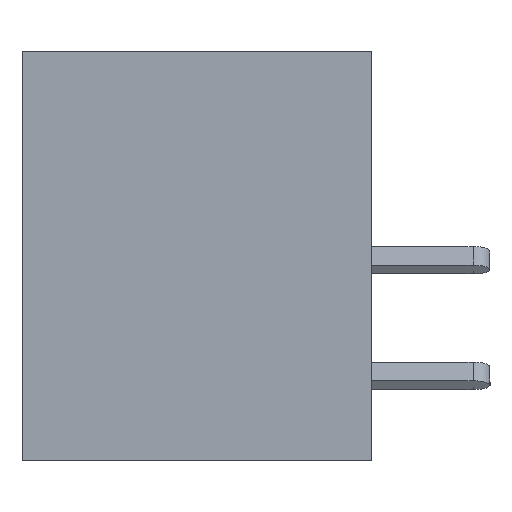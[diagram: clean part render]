
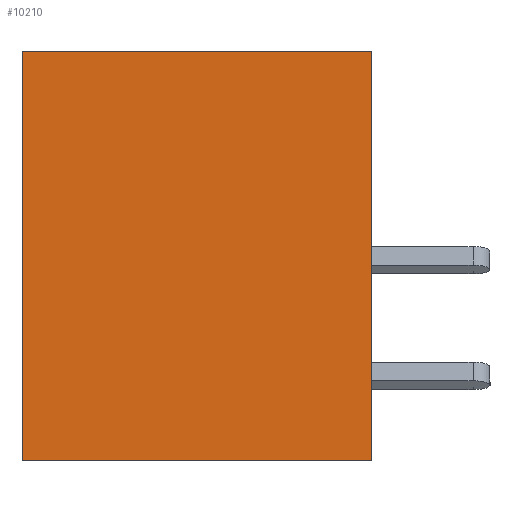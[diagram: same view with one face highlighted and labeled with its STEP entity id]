
A CAD part, left-side view. The second image highlights one B-rep face of the part: STEP entity #10210.
In plain terms, the highlighted planar face has unit normal (-1, 0, 0).
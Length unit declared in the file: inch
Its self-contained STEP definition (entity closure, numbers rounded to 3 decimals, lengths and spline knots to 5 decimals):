
#435 = VERTEX_POINT ( 'NONE', #22422 ) ;
#502 = CARTESIAN_POINT ( 'NONE',  ( 0., 0.453, 0. ) ) ;
#1654 = VECTOR ( 'NONE', #20604, 39.37008 ) ;
#2089 = DIRECTION ( 'NONE',  ( 0., 0., 1. ) ) ;
#2254 = CARTESIAN_POINT ( 'NONE',  ( 0., 0.453, 0. ) ) ;
#2281 = EDGE_CURVE ( 'NONE', #12305, #7209, #14896, .T. ) ;
#3637 = CARTESIAN_POINT ( 'NONE',  ( 0., 0.453, 0. ) ) ;
#3675 = VECTOR ( 'NONE', #17162, 39.37008 ) ;
#4034 = EDGE_CURVE ( 'NONE', #7209, #435, #6581, .T. ) ;
#5553 = DIRECTION ( 'NONE',  ( 0., 0., -1. ) ) ;
#6581 = LINE ( 'NONE', #19888, #15384 ) ;
#7209 = VERTEX_POINT ( 'NONE', #13214 ) ;
#7960 = ORIENTED_EDGE ( 'NONE', *, *, #4034, .T. ) ;
#9922 = EDGE_LOOP ( 'NONE', ( #7960, #14663, #12799, #20700 ) ) ;
#10210 = ADVANCED_FACE ( 'NONE', ( #11950 ), #14912, .F. ) ;
#10369 = VERTEX_POINT ( 'NONE', #14767 ) ;
#11029 = EDGE_CURVE ( 'NONE', #12305, #10369, #14261, .T. ) ;
#11950 = FACE_OUTER_BOUND ( 'NONE', #9922, .T. ) ;
#12305 = VERTEX_POINT ( 'NONE', #23665 ) ;
#12799 = ORIENTED_EDGE ( 'NONE', *, *, #11029, .F. ) ;
#13196 = CARTESIAN_POINT ( 'NONE',  ( 0., 0.453, -0.531 ) ) ;
#13214 = CARTESIAN_POINT ( 'NONE',  ( 0., 0., -0.531 ) ) ;
#14261 = LINE ( 'NONE', #2254, #21632 ) ;
#14663 = ORIENTED_EDGE ( 'NONE', *, *, #23825, .F. ) ;
#14767 = CARTESIAN_POINT ( 'NONE',  ( 0., 0.453, 0. ) ) ;
#14896 = LINE ( 'NONE', #13196, #1654 ) ;
#14912 = PLANE ( 'NONE',  #19265 ) ;
#15384 = VECTOR ( 'NONE', #16343, 39.37008 ) ;
#16343 = DIRECTION ( 'NONE',  ( 0., 0., 1. ) ) ;
#16781 = DIRECTION ( 'NONE',  ( 1., 0., 0. ) ) ;
#17162 = DIRECTION ( 'NONE',  ( 0., -1., 0. ) ) ;
#19265 = AXIS2_PLACEMENT_3D ( 'NONE', #3637, #16781, #5553 ) ;
#19850 = LINE ( 'NONE', #502, #3675 ) ;
#19888 = CARTESIAN_POINT ( 'NONE',  ( 0., 0., 0. ) ) ;
#20604 = DIRECTION ( 'NONE',  ( 0., -1., 0. ) ) ;
#20700 = ORIENTED_EDGE ( 'NONE', *, *, #2281, .T. ) ;
#21632 = VECTOR ( 'NONE', #2089, 39.37008 ) ;
#22422 = CARTESIAN_POINT ( 'NONE',  ( 0., 0., 0. ) ) ;
#23665 = CARTESIAN_POINT ( 'NONE',  ( 0., 0.453, -0.531 ) ) ;
#23825 = EDGE_CURVE ( 'NONE', #10369, #435, #19850, .T. ) ;
